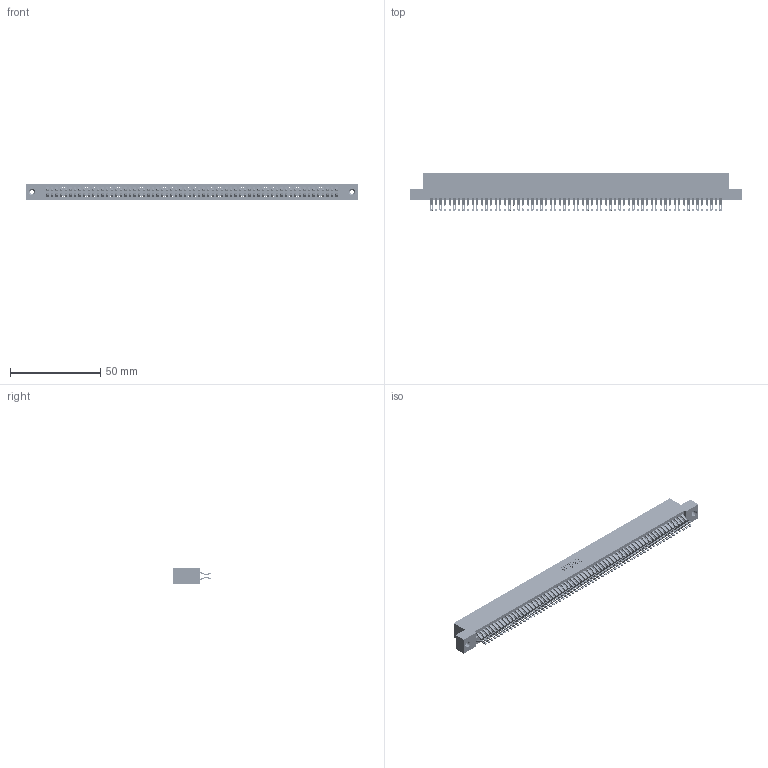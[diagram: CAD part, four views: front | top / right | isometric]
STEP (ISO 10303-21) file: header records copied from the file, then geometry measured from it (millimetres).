
FILE_DESCRIPTION (( 'STEP AP203' ), '1' );
FILE_NAME ('345-128-555-208.STEP', '2018-10-19T21:10:15', ( '' ), ( '' ), 'SwSTEP 2.0', 'SolidWorks 2016', '' );
FILE_SCHEMA (( 'CONFIG_CONTROL_DESIGN' ));
Length unit declared in the file: inch
Products named in the file (4): 345 Part_Flush Mounting Lugs - 0.156 Dia-TI; 345-128-555-208; 345-250-001_345-250-003-102; 345-292-001_555 Tail
Assembly tree (131 placements, depth 2):
  345-128-555-208
    345 Part_Flush Mounting Lugs - 0.156 Dia-TI
    345-292-001_555 Tail  x128
    345-250-001_345-250-003-102  x2
Bounding box: 183.77 x 21.13 x 9.4 mm (x, y, z)
Volume: 18420.5 mm3; surface area: 28959.4 mm2
Topology: 131 solids, 131 shells, 7354 faces, 23133 edges, 15414 vertices
Faces by surface type: plane 4080, cylinder 3258, cone 12, torus 4
Entity records: 48766 total; most frequent: CARTESIAN_POINT 8169, ORIENTED_EDGE 8066, DIRECTION 7171, EDGE_CURVE 4033, VECTOR 3605, LINE 3605, VERTEX_POINT 2684, AXIS2_PLACEMENT_3D 1783
